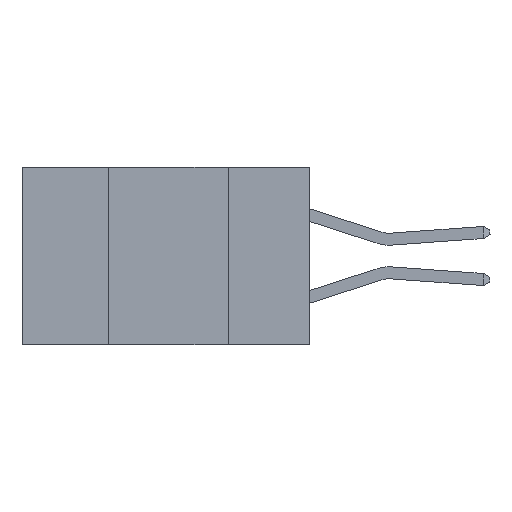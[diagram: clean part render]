
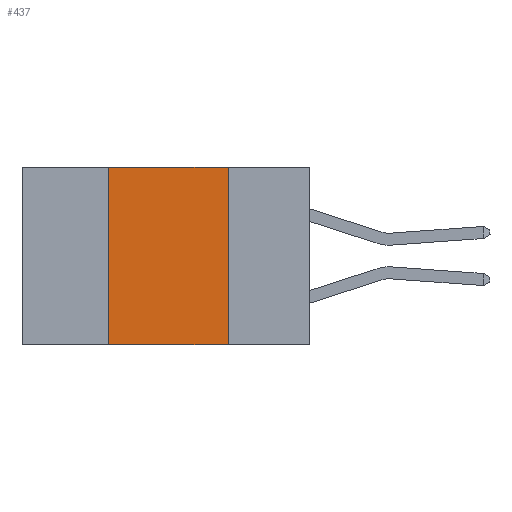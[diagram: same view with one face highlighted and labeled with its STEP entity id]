
A CAD part, left-side view. The second image highlights one B-rep face of the part: STEP entity #437.
In plain terms, the highlighted planar face has unit normal (-1, 0, 0).
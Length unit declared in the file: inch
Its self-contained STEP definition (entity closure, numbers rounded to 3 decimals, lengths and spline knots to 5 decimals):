
#137 = LINE ( 'NONE', #2210, #7635 ) ;
#379 = EDGE_CURVE ( 'NONE', #8515, #7568, #3611, .T. ) ;
#437 = ADVANCED_FACE ( 'NONE', ( #1754 ), #8413, .F. ) ;
#974 = DIRECTION ( 'NONE',  ( 0., 0., -1. ) ) ;
#1167 = EDGE_CURVE ( 'NONE', #8515, #6785, #137, .T. ) ;
#1169 = EDGE_CURVE ( 'NONE', #6785, #2682, #4033, .T. ) ;
#1188 = CARTESIAN_POINT ( 'NONE',  ( 0., 0.17, -0.37 ) ) ;
#1199 = EDGE_CURVE ( 'NONE', #2682, #7568, #3808, .T. ) ;
#1610 = DIRECTION ( 'NONE',  ( 0., -1., 0. ) ) ;
#1754 = FACE_OUTER_BOUND ( 'NONE', #3246, .T. ) ;
#1849 = VECTOR ( 'NONE', #974, 39.37008 ) ;
#2210 = CARTESIAN_POINT ( 'NONE',  ( 0., 0.42, -0.37 ) ) ;
#2370 = ORIENTED_EDGE ( 'NONE', *, *, #1199, .F. ) ;
#2682 = VERTEX_POINT ( 'NONE', #6641 ) ;
#3246 = EDGE_LOOP ( 'NONE', ( #2370, #4504, #6979, #5602 ) ) ;
#3611 = LINE ( 'NONE', #4144, #8188 ) ;
#3808 = LINE ( 'NONE', #5895, #1849 ) ;
#3988 = CARTESIAN_POINT ( 'NONE',  ( 0., 0.6, 0. ) ) ;
#4033 = LINE ( 'NONE', #3988, #8054 ) ;
#4144 = CARTESIAN_POINT ( 'NONE',  ( 0., 0.6, -0.37 ) ) ;
#4504 = ORIENTED_EDGE ( 'NONE', *, *, #1169, .F. ) ;
#5217 = CARTESIAN_POINT ( 'NONE',  ( 0., 0.42, -0.37 ) ) ;
#5602 = ORIENTED_EDGE ( 'NONE', *, *, #379, .T. ) ;
#5895 = CARTESIAN_POINT ( 'NONE',  ( 0., 0.17, -0.37 ) ) ;
#6641 = CARTESIAN_POINT ( 'NONE',  ( 0., 0.17, 0. ) ) ;
#6763 = CARTESIAN_POINT ( 'NONE',  ( 0., 0.6, 0. ) ) ;
#6785 = VERTEX_POINT ( 'NONE', #7567 ) ;
#6979 = ORIENTED_EDGE ( 'NONE', *, *, #1167, .F. ) ;
#7151 = DIRECTION ( 'NONE',  ( 0., -1., 0. ) ) ;
#7486 = DIRECTION ( 'NONE',  ( 1., 0., 0. ) ) ;
#7567 = CARTESIAN_POINT ( 'NONE',  ( 0., 0.42, 0. ) ) ;
#7568 = VERTEX_POINT ( 'NONE', #1188 ) ;
#7635 = VECTOR ( 'NONE', #7815, 39.37008 ) ;
#7815 = DIRECTION ( 'NONE',  ( 0., 0., 1. ) ) ;
#8054 = VECTOR ( 'NONE', #1610, 39.37008 ) ;
#8188 = VECTOR ( 'NONE', #7151, 39.37008 ) ;
#8413 = PLANE ( 'NONE',  #8445 ) ;
#8445 = AXIS2_PLACEMENT_3D ( 'NONE', #6763, #7486, #8720 ) ;
#8515 = VERTEX_POINT ( 'NONE', #5217 ) ;
#8720 = DIRECTION ( 'NONE',  ( 0., 0., -1. ) ) ;
